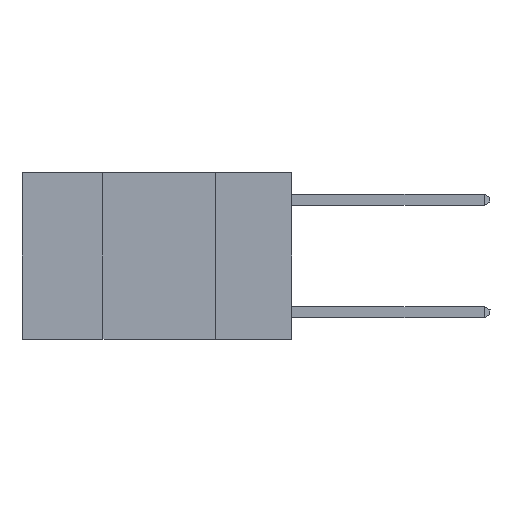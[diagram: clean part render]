
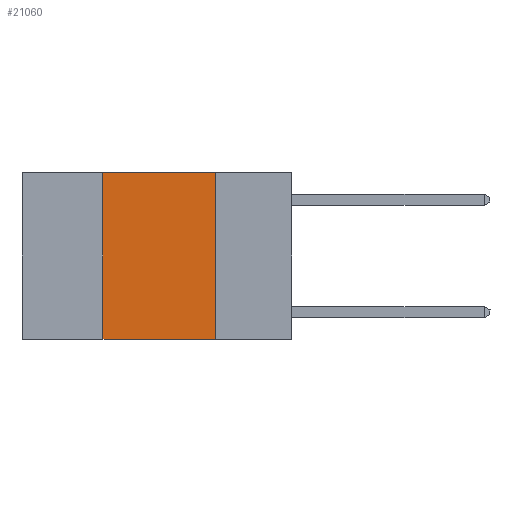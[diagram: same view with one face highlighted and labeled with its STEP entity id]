
A CAD part, left-side view. The second image highlights one B-rep face of the part: STEP entity #21060.
In plain terms, the highlighted planar face has unit normal (-1, 0, 0).
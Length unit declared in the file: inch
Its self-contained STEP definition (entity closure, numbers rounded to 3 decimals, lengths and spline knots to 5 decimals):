
#771 = ORIENTED_EDGE ( 'NONE', *, *, #14212, .F. ) ;
#1329 = DIRECTION ( 'NONE',  ( 0., 0., -1. ) ) ;
#2468 = ORIENTED_EDGE ( 'NONE', *, *, #16182, .F. ) ;
#2795 = DIRECTION ( 'NONE',  ( 1., 0., 0. ) ) ;
#3398 = VERTEX_POINT ( 'NONE', #9659 ) ;
#4005 = CARTESIAN_POINT ( 'NONE',  ( 0., 0.17, 0. ) ) ;
#4240 = ORIENTED_EDGE ( 'NONE', *, *, #20700, .T. ) ;
#4891 = FACE_OUTER_BOUND ( 'NONE', #25950, .T. ) ;
#6820 = ORIENTED_EDGE ( 'NONE', *, *, #8350, .F. ) ;
#7995 = CARTESIAN_POINT ( 'NONE',  ( 0., 0.42, 0. ) ) ;
#8350 = EDGE_CURVE ( 'NONE', #19357, #19266, #26029, .T. ) ;
#8449 = DIRECTION ( 'NONE',  ( 0., -1., 0. ) ) ;
#8956 = CARTESIAN_POINT ( 'NONE',  ( 0., 0.42, 0. ) ) ;
#9247 = VECTOR ( 'NONE', #20448, 39.37008 ) ;
#9659 = CARTESIAN_POINT ( 'NONE',  ( 0., 0.42, -0.37 ) ) ;
#12098 = PLANE ( 'NONE',  #21993 ) ;
#13032 = LINE ( 'NONE', #8956, #25528 ) ;
#14212 = EDGE_CURVE ( 'NONE', #3398, #26795, #13032, .T. ) ;
#16182 = EDGE_CURVE ( 'NONE', #26795, #19357, #22470, .T. ) ;
#16783 = CARTESIAN_POINT ( 'NONE',  ( 0., 0.6, 0. ) ) ;
#17806 = CARTESIAN_POINT ( 'NONE',  ( 0., 0.17, 0. ) ) ;
#18085 = CARTESIAN_POINT ( 'NONE',  ( 0., 0.6, 0. ) ) ;
#19176 = DIRECTION ( 'NONE',  ( 0., 0., -1. ) ) ;
#19266 = VERTEX_POINT ( 'NONE', #24825 ) ;
#19357 = VERTEX_POINT ( 'NONE', #4005 ) ;
#20448 = DIRECTION ( 'NONE',  ( 0., -1., 0. ) ) ;
#20700 = EDGE_CURVE ( 'NONE', #3398, #19266, #21431, .T. ) ;
#21060 = ADVANCED_FACE ( 'NONE', ( #4891 ), #12098, .F. ) ;
#21431 = LINE ( 'NONE', #29571, #22173 ) ;
#21993 = AXIS2_PLACEMENT_3D ( 'NONE', #16783, #2795, #19176 ) ;
#22173 = VECTOR ( 'NONE', #8449, 39.37008 ) ;
#22470 = LINE ( 'NONE', #18085, #9247 ) ;
#24825 = CARTESIAN_POINT ( 'NONE',  ( 0., 0.17, -0.37 ) ) ;
#25306 = VECTOR ( 'NONE', #1329, 39.37008 ) ;
#25528 = VECTOR ( 'NONE', #30181, 39.37008 ) ;
#25950 = EDGE_LOOP ( 'NONE', ( #6820, #2468, #771, #4240 ) ) ;
#26029 = LINE ( 'NONE', #17806, #25306 ) ;
#26795 = VERTEX_POINT ( 'NONE', #7995 ) ;
#29571 = CARTESIAN_POINT ( 'NONE',  ( 0., 0.6, -0.37 ) ) ;
#30181 = DIRECTION ( 'NONE',  ( 0., 0., 1. ) ) ;
